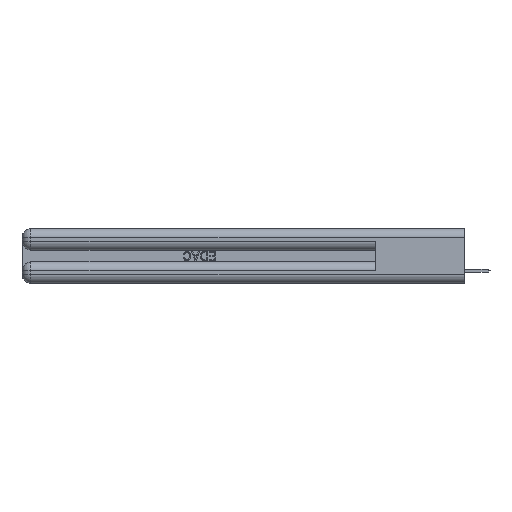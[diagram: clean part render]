
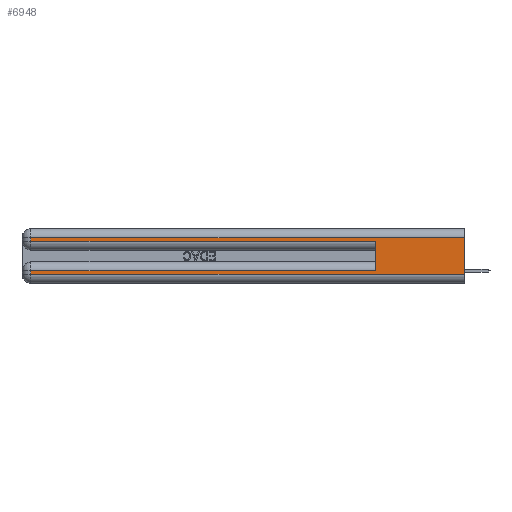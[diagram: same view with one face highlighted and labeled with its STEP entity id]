
A CAD part, left-side view. The second image highlights one B-rep face of the part: STEP entity #6948.
In plain terms, the highlighted planar face has unit normal (-1, 0, 0).
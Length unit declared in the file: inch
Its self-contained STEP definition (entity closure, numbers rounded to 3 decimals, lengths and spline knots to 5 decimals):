
#451 = FACE_OUTER_BOUND ( 'NONE', #36213, .T. ) ;
#456 = CARTESIAN_POINT ( 'NONE',  ( 0., 0.6, 0.085 ) ) ;
#1029 = EDGE_CURVE ( 'NONE', #3889, #41340, #42412, .T. ) ;
#1830 = VECTOR ( 'NONE', #5168, 39.37008 ) ;
#2425 = CARTESIAN_POINT ( 'NONE',  ( 0., 0.6, 0.285 ) ) ;
#2888 = ORIENTED_EDGE ( 'NONE', *, *, #42959, .T. ) ;
#3376 = DIRECTION ( 'NONE',  ( 0., 0., -1. ) ) ;
#3391 = VERTEX_POINT ( 'NONE', #35107 ) ;
#3617 = LINE ( 'NONE', #29812, #20285 ) ;
#3781 = CARTESIAN_POINT ( 'NONE',  ( 0., 2.94, 0.285 ) ) ;
#3889 = VERTEX_POINT ( 'NONE', #24745 ) ;
#4048 = CARTESIAN_POINT ( 'NONE',  ( 0., 0., 0.37 ) ) ;
#4257 = CARTESIAN_POINT ( 'NONE',  ( 0., 0., 0.06 ) ) ;
#4469 = DIRECTION ( 'NONE',  ( 0., 1., 0. ) ) ;
#4554 = VERTEX_POINT ( 'NONE', #456 ) ;
#5114 = EDGE_CURVE ( 'NONE', #14225, #8776, #23077, .T. ) ;
#5168 = DIRECTION ( 'NONE',  ( 0., 1., 0. ) ) ;
#6905 = LINE ( 'NONE', #20895, #40690 ) ;
#6948 = ADVANCED_FACE ( 'NONE', ( #451 ), #34389, .F. ) ;
#8574 = DIRECTION ( 'NONE',  ( 0., 0., 1. ) ) ;
#8776 = VERTEX_POINT ( 'NONE', #40323 ) ;
#9552 = AXIS2_PLACEMENT_3D ( 'NONE', #4048, #30754, #17826 ) ;
#9602 = EDGE_CURVE ( 'NONE', #3391, #3889, #42951, .T. ) ;
#9852 = LINE ( 'NONE', #35224, #39477 ) ;
#12799 = EDGE_CURVE ( 'NONE', #41340, #26953, #22440, .T. ) ;
#12911 = CARTESIAN_POINT ( 'NONE',  ( 0., 0., 0.285 ) ) ;
#13164 = VERTEX_POINT ( 'NONE', #4257 ) ;
#14195 = VECTOR ( 'NONE', #19686, 39.37008 ) ;
#14225 = VERTEX_POINT ( 'NONE', #15109 ) ;
#15109 = CARTESIAN_POINT ( 'NONE',  ( 0., 2.94, 0.085 ) ) ;
#15286 = ORIENTED_EDGE ( 'NONE', *, *, #41249, .F. ) ;
#15907 = CARTESIAN_POINT ( 'NONE',  ( 0., 2.94, 0.37 ) ) ;
#17826 = DIRECTION ( 'NONE',  ( 0., 0., -1. ) ) ;
#18846 = DIRECTION ( 'NONE',  ( 0., -1., 0. ) ) ;
#18859 = ORIENTED_EDGE ( 'NONE', *, *, #5114, .T. ) ;
#19686 = DIRECTION ( 'NONE',  ( 0., 0., -1. ) ) ;
#19755 = ORIENTED_EDGE ( 'NONE', *, *, #29765, .T. ) ;
#20285 = VECTOR ( 'NONE', #3376, 39.37008 ) ;
#20653 = CARTESIAN_POINT ( 'NONE',  ( 0., 2.94, 0.37 ) ) ;
#20895 = CARTESIAN_POINT ( 'NONE',  ( 0., 0., 0.085 ) ) ;
#22440 = LINE ( 'NONE', #12911, #33333 ) ;
#22696 = ORIENTED_EDGE ( 'NONE', *, *, #1029, .T. ) ;
#23077 = LINE ( 'NONE', #20653, #14195 ) ;
#24745 = CARTESIAN_POINT ( 'NONE',  ( 0., 2.94, 0.31 ) ) ;
#26868 = ORIENTED_EDGE ( 'NONE', *, *, #12799, .T. ) ;
#26953 = VERTEX_POINT ( 'NONE', #2425 ) ;
#29765 = EDGE_CURVE ( 'NONE', #4554, #14225, #6905, .T. ) ;
#29812 = CARTESIAN_POINT ( 'NONE',  ( 0., 0., 0.37 ) ) ;
#30585 = LINE ( 'NONE', #42140, #35800 ) ;
#30754 = DIRECTION ( 'NONE',  ( 1., 0., 0. ) ) ;
#31420 = VECTOR ( 'NONE', #36075, 39.37008 ) ;
#33333 = VECTOR ( 'NONE', #39504, 39.37008 ) ;
#33530 = ORIENTED_EDGE ( 'NONE', *, *, #41662, .F. ) ;
#34389 = PLANE ( 'NONE',  #9552 ) ;
#35107 = CARTESIAN_POINT ( 'NONE',  ( 0., 0., 0.31 ) ) ;
#35224 = CARTESIAN_POINT ( 'NONE',  ( 0., 0., 0.06 ) ) ;
#35800 = VECTOR ( 'NONE', #8574, 39.37008 ) ;
#35977 = ORIENTED_EDGE ( 'NONE', *, *, #9602, .T. ) ;
#36075 = DIRECTION ( 'NONE',  ( 0., 0., -1. ) ) ;
#36213 = EDGE_LOOP ( 'NONE', ( #15286, #35977, #22696, #26868, #33530, #19755, #18859, #2888 ) ) ;
#39477 = VECTOR ( 'NONE', #18846, 39.37008 ) ;
#39504 = DIRECTION ( 'NONE',  ( 0., -1., 0. ) ) ;
#40323 = CARTESIAN_POINT ( 'NONE',  ( 0., 2.94, 0.06 ) ) ;
#40690 = VECTOR ( 'NONE', #4469, 39.37008 ) ;
#41249 = EDGE_CURVE ( 'NONE', #3391, #13164, #3617, .T. ) ;
#41340 = VERTEX_POINT ( 'NONE', #3781 ) ;
#41510 = CARTESIAN_POINT ( 'NONE',  ( 0., 0., 0.31 ) ) ;
#41662 = EDGE_CURVE ( 'NONE', #4554, #26953, #30585, .T. ) ;
#42140 = CARTESIAN_POINT ( 'NONE',  ( 0., 0.6, 0.145 ) ) ;
#42412 = LINE ( 'NONE', #15907, #31420 ) ;
#42951 = LINE ( 'NONE', #41510, #1830 ) ;
#42959 = EDGE_CURVE ( 'NONE', #8776, #13164, #9852, .T. ) ;
